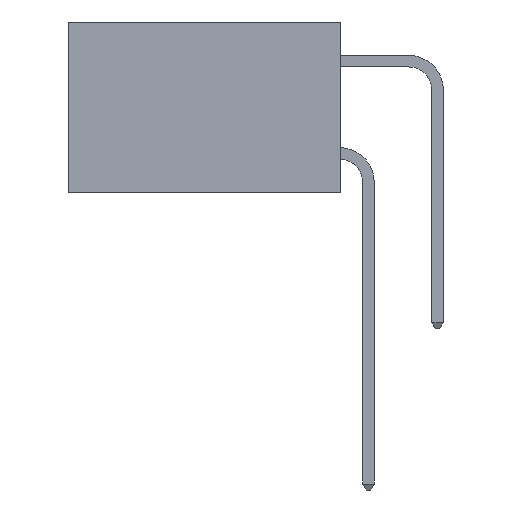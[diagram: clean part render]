
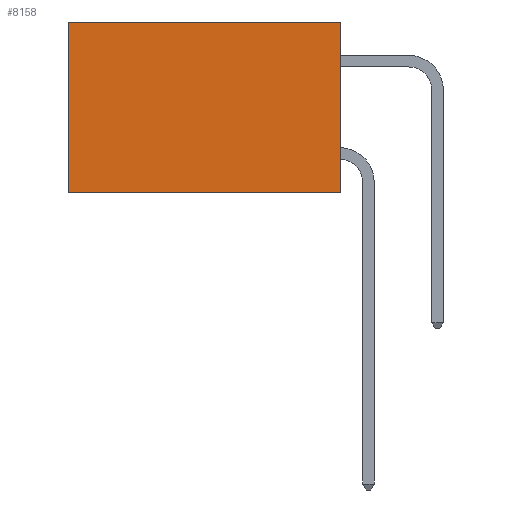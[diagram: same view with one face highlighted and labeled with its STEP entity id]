
A CAD part, left-side view. The second image highlights one B-rep face of the part: STEP entity #8158.
In plain terms, the highlighted planar face has unit normal (-1, 0, 0).
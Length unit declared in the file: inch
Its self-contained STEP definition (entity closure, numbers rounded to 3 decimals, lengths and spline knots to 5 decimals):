
#138 = FACE_OUTER_BOUND ( 'NONE', #1844, .T. ) ;
#510 = LINE ( 'NONE', #2633, #6685 ) ;
#1097 = DIRECTION ( 'NONE',  ( 0., 0., -1. ) ) ;
#1163 = ORIENTED_EDGE ( 'NONE', *, *, #2294, .T. ) ;
#1303 = VECTOR ( 'NONE', #5868, 39.37008 ) ;
#1844 = EDGE_LOOP ( 'NONE', ( #1163, #3555, #8140, #6229 ) ) ;
#2062 = EDGE_CURVE ( 'NONE', #2912, #6101, #9765, .T. ) ;
#2294 = EDGE_CURVE ( 'NONE', #6937, #6101, #3437, .T. ) ;
#2464 = CARTESIAN_POINT ( 'NONE',  ( 0.277, 0., -0.37 ) ) ;
#2607 = LINE ( 'NONE', #7794, #6696 ) ;
#2633 = CARTESIAN_POINT ( 'NONE',  ( 0.277, 0., -0.37 ) ) ;
#2912 = VERTEX_POINT ( 'NONE', #2464 ) ;
#3437 = LINE ( 'NONE', #6039, #1303 ) ;
#3555 = ORIENTED_EDGE ( 'NONE', *, *, #2062, .F. ) ;
#3752 = EDGE_CURVE ( 'NONE', #6926, #6937, #2607, .T. ) ;
#4192 = EDGE_CURVE ( 'NONE', #6926, #2912, #510, .T. ) ;
#4211 = PLANE ( 'NONE',  #4448 ) ;
#4448 = AXIS2_PLACEMENT_3D ( 'NONE', #6621, #9866, #5009 ) ;
#4919 = CARTESIAN_POINT ( 'NONE',  ( 0.277, 0.59, -0.37 ) ) ;
#5009 = DIRECTION ( 'NONE',  ( 0., 0., -1. ) ) ;
#5026 = CARTESIAN_POINT ( 'NONE',  ( 0.277, 0.59, 0. ) ) ;
#5868 = DIRECTION ( 'NONE',  ( 0., 0., -1. ) ) ;
#6039 = CARTESIAN_POINT ( 'NONE',  ( 0.277, 0.59, -0.37 ) ) ;
#6101 = VERTEX_POINT ( 'NONE', #4919 ) ;
#6229 = ORIENTED_EDGE ( 'NONE', *, *, #3752, .T. ) ;
#6621 = CARTESIAN_POINT ( 'NONE',  ( 0.277, 0., -0.37 ) ) ;
#6685 = VECTOR ( 'NONE', #1097, 39.37008 ) ;
#6696 = VECTOR ( 'NONE', #8393, 39.37008 ) ;
#6926 = VERTEX_POINT ( 'NONE', #8307 ) ;
#6937 = VERTEX_POINT ( 'NONE', #5026 ) ;
#7574 = DIRECTION ( 'NONE',  ( 0., 1., 0. ) ) ;
#7634 = VECTOR ( 'NONE', #7574, 39.37008 ) ;
#7683 = CARTESIAN_POINT ( 'NONE',  ( 0.277, 0., -0.37 ) ) ;
#7794 = CARTESIAN_POINT ( 'NONE',  ( 0.277, 0., 0. ) ) ;
#8140 = ORIENTED_EDGE ( 'NONE', *, *, #4192, .F. ) ;
#8158 = ADVANCED_FACE ( 'NONE', ( #138 ), #4211, .F. ) ;
#8307 = CARTESIAN_POINT ( 'NONE',  ( 0.277, 0., 0. ) ) ;
#8393 = DIRECTION ( 'NONE',  ( 0., 1., 0. ) ) ;
#9765 = LINE ( 'NONE', #7683, #7634 ) ;
#9866 = DIRECTION ( 'NONE',  ( 1., 0., 0. ) ) ;
